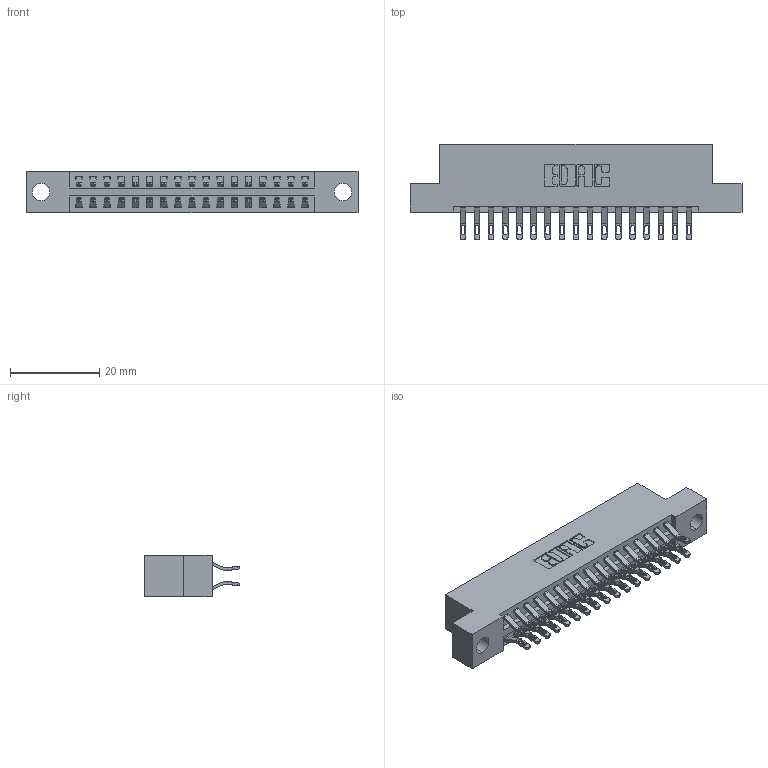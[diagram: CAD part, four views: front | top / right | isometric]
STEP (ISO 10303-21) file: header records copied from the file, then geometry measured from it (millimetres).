
FILE_DESCRIPTION (( 'STEP AP203' ), '1' );
FILE_NAME ('346-034-555-204.STEP', '2022-05-19T20:00:43', ( '' ), ( '' ), 'SwSTEP 2.0', 'SolidWorks 2020', '' );
FILE_SCHEMA (( 'CONFIG_CONTROL_DESIGN' ));
Length unit declared in the file: inch
Products named in the file (3): 345-292-001_555 Tail; 346-034-555-204; 346 Part_Flush Mounting Lugs - 0.156 Dia-TH
Assembly tree (35 placements, depth 2):
  346-034-555-204
    346 Part_Flush Mounting Lugs - 0.156 Dia-TH
    345-292-001_555 Tail  x34
Bounding box: 74.55 x 21.46 x 9.4 mm (x, y, z)
Volume: 7068 mm3; surface area: 9521.9 mm2
Topology: 35 solids, 35 shells, 2108 faces, 6587 edges, 4390 vertices
Faces by surface type: plane 1212, cylinder 896
Entity records: 15205 total; most frequent: CARTESIAN_POINT 2580, ORIENTED_EDGE 2482, DIRECTION 2293, EDGE_CURVE 1241, VECTOR 1021, LINE 1021, VERTEX_POINT 826, AXIS2_PLACEMENT_3D 636
